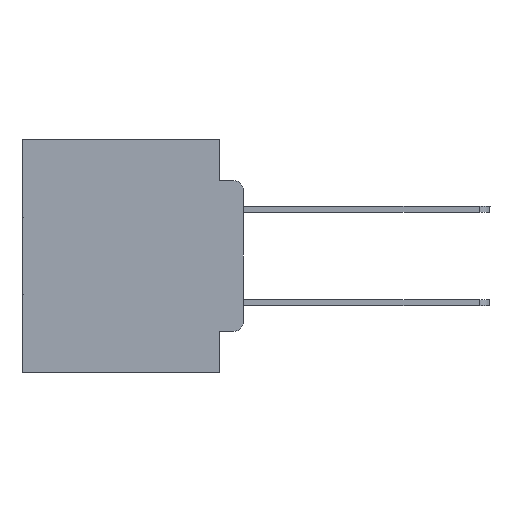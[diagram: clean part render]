
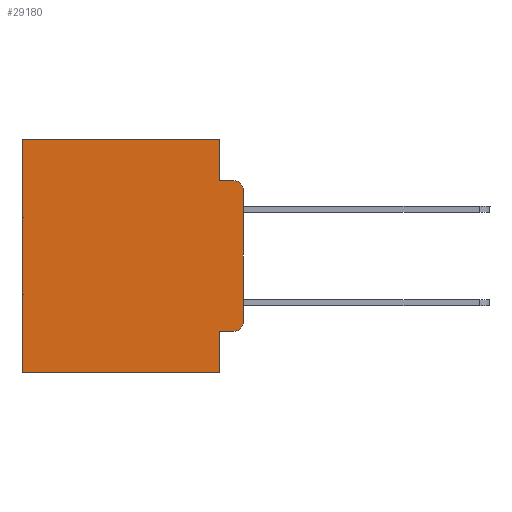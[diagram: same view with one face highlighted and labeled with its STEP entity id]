
A CAD part, left-side view. The second image highlights one B-rep face of the part: STEP entity #29180.
In plain terms, the highlighted planar face has unit normal (-1, 0, 0).
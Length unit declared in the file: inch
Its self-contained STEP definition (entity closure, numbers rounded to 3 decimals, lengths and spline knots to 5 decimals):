
#58 = DIRECTION ( 'NONE',  ( 0., 0., -1. ) ) ;
#257 = DIRECTION ( 'NONE',  ( 0., 1., 0. ) ) ;
#299 = ORIENTED_EDGE ( 'NONE', *, *, #24227, .F. ) ;
#1628 = CARTESIAN_POINT ( 'NONE',  ( 0.298, 0.02, -0.1085 ) ) ;
#1682 = CARTESIAN_POINT ( 'NONE',  ( 0.298, 0.051, 0. ) ) ;
#1748 = CARTESIAN_POINT ( 'NONE',  ( 0.298, 0., 0. ) ) ;
#1788 = VERTEX_POINT ( 'NONE', #27223 ) ;
#1991 = AXIS2_PLACEMENT_3D ( 'NONE', #17054, #2778, #19392 ) ;
#2778 = DIRECTION ( 'NONE',  ( 1., 0., 0. ) ) ;
#2850 = EDGE_CURVE ( 'NONE', #10158, #25653, #5569, .T. ) ;
#3257 = CARTESIAN_POINT ( 'NONE',  ( 0.298, 0.051, 0. ) ) ;
#3465 = ORIENTED_EDGE ( 'NONE', *, *, #28963, .T. ) ;
#3850 = VECTOR ( 'NONE', #14404, 39.37008 ) ;
#4070 = DIRECTION ( 'NONE',  ( 0., 0., -1. ) ) ;
#4407 = LINE ( 'NONE', #3257, #10001 ) ;
#4523 = ORIENTED_EDGE ( 'NONE', *, *, #12392, .T. ) ;
#4954 = EDGE_CURVE ( 'NONE', #16373, #14156, #12520, .T. ) ;
#5569 = LINE ( 'NONE', #10298, #28255 ) ;
#6296 = VERTEX_POINT ( 'NONE', #1682 ) ;
#6715 = FACE_OUTER_BOUND ( 'NONE', #25470, .T. ) ;
#7340 = VECTOR ( 'NONE', #257, 39.37008 ) ;
#9266 = CARTESIAN_POINT ( 'NONE',  ( 0.298, 0.473, -0.5 ) ) ;
#10001 = VECTOR ( 'NONE', #15132, 39.37008 ) ;
#10158 = VERTEX_POINT ( 'NONE', #15834 ) ;
#10298 = CARTESIAN_POINT ( 'NONE',  ( 0.298, 0., -0.5 ) ) ;
#10352 = AXIS2_PLACEMENT_3D ( 'NONE', #1628, #18269, #4070 ) ;
#10503 = VERTEX_POINT ( 'NONE', #22981 ) ;
#10526 = CIRCLE ( 'NONE', #27108, 0.02 ) ;
#11140 = VERTEX_POINT ( 'NONE', #15995 ) ;
#11297 = CARTESIAN_POINT ( 'NONE',  ( 0.298, 0.02, -0.0885 ) ) ;
#11565 = CARTESIAN_POINT ( 'NONE',  ( 0.298, 0.02, -0.3915 ) ) ;
#11865 = VECTOR ( 'NONE', #16343, 39.37008 ) ;
#12013 = CARTESIAN_POINT ( 'NONE',  ( 0.298, 0.051, -0.0885 ) ) ;
#12392 = EDGE_CURVE ( 'NONE', #1788, #14156, #10526, .T. ) ;
#12520 = LINE ( 'NONE', #1748, #23510 ) ;
#13088 = ORIENTED_EDGE ( 'NONE', *, *, #21128, .F. ) ;
#13953 = DIRECTION ( 'NONE',  ( 0., 0., -1. ) ) ;
#13965 = CARTESIAN_POINT ( 'NONE',  ( 0.298, 0.473, 0. ) ) ;
#14156 = VERTEX_POINT ( 'NONE', #27448 ) ;
#14404 = DIRECTION ( 'NONE',  ( 0., -1., 0. ) ) ;
#14896 = VERTEX_POINT ( 'NONE', #11297 ) ;
#14963 = ORIENTED_EDGE ( 'NONE', *, *, #22366, .T. ) ;
#15132 = DIRECTION ( 'NONE',  ( 0., 0., -1. ) ) ;
#15834 = CARTESIAN_POINT ( 'NONE',  ( 0.298, 0.051, -0.5 ) ) ;
#15995 = CARTESIAN_POINT ( 'NONE',  ( 0.298, 0.473, 0. ) ) ;
#16033 = ORIENTED_EDGE ( 'NONE', *, *, #23197, .T. ) ;
#16343 = DIRECTION ( 'NONE',  ( 0., 0., -1. ) ) ;
#16373 = VERTEX_POINT ( 'NONE', #27255 ) ;
#17054 = CARTESIAN_POINT ( 'NONE',  ( 0.298, 0., 0. ) ) ;
#17141 = ORIENTED_EDGE ( 'NONE', *, *, #18515, .F. ) ;
#17356 = LINE ( 'NONE', #19565, #28956 ) ;
#17665 = CARTESIAN_POINT ( 'NONE',  ( 0.298, 0.051, -0.4115 ) ) ;
#17792 = VERTEX_POINT ( 'NONE', #28579 ) ;
#18269 = DIRECTION ( 'NONE',  ( -1., 0., 0. ) ) ;
#18515 = EDGE_CURVE ( 'NONE', #17792, #10158, #17356, .T. ) ;
#19124 = LINE ( 'NONE', #21671, #7340 ) ;
#19296 = PLANE ( 'NONE',  #1991 ) ;
#19392 = DIRECTION ( 'NONE',  ( 0., 0., -1. ) ) ;
#19565 = CARTESIAN_POINT ( 'NONE',  ( 0.298, 0.051, 0. ) ) ;
#20011 = DIRECTION ( 'NONE',  ( 0., -1., 0. ) ) ;
#21128 = EDGE_CURVE ( 'NONE', #6296, #10503, #4407, .T. ) ;
#21671 = CARTESIAN_POINT ( 'NONE',  ( 0.298, 0., 0. ) ) ;
#21901 = DIRECTION ( 'NONE',  ( 0., 0., -1. ) ) ;
#22366 = EDGE_CURVE ( 'NONE', #6296, #11140, #19124, .T. ) ;
#22751 = LINE ( 'NONE', #17665, #26651 ) ;
#22981 = CARTESIAN_POINT ( 'NONE',  ( 0.298, 0.051, -0.0885 ) ) ;
#23197 = EDGE_CURVE ( 'NONE', #17792, #1788, #22751, .T. ) ;
#23510 = VECTOR ( 'NONE', #58, 39.37008 ) ;
#23727 = CIRCLE ( 'NONE', #10352, 0.02 ) ;
#24227 = EDGE_CURVE ( 'NONE', #10503, #14896, #29548, .T. ) ;
#24848 = EDGE_CURVE ( 'NONE', #16373, #14896, #23727, .T. ) ;
#25470 = EDGE_LOOP ( 'NONE', ( #26908, #29201, #299, #13088, #14963, #3465, #27732, #17141, #16033, #4523 ) ) ;
#25653 = VERTEX_POINT ( 'NONE', #9266 ) ;
#25850 = DIRECTION ( 'NONE',  ( 0., 1., 0. ) ) ;
#26651 = VECTOR ( 'NONE', #20011, 39.37008 ) ;
#26908 = ORIENTED_EDGE ( 'NONE', *, *, #4954, .F. ) ;
#27108 = AXIS2_PLACEMENT_3D ( 'NONE', #11565, #27870, #13953 ) ;
#27223 = CARTESIAN_POINT ( 'NONE',  ( 0.298, 0.02, -0.4115 ) ) ;
#27255 = CARTESIAN_POINT ( 'NONE',  ( 0.298, 0., -0.1085 ) ) ;
#27448 = CARTESIAN_POINT ( 'NONE',  ( 0.298, 0., -0.3915 ) ) ;
#27732 = ORIENTED_EDGE ( 'NONE', *, *, #2850, .F. ) ;
#27870 = DIRECTION ( 'NONE',  ( -1., 0., 0. ) ) ;
#28255 = VECTOR ( 'NONE', #25850, 39.37008 ) ;
#28579 = CARTESIAN_POINT ( 'NONE',  ( 0.298, 0.051, -0.4115 ) ) ;
#28956 = VECTOR ( 'NONE', #21901, 39.37008 ) ;
#28963 = EDGE_CURVE ( 'NONE', #11140, #25653, #30413, .T. ) ;
#29180 = ADVANCED_FACE ( 'NONE', ( #6715 ), #19296, .F. ) ;
#29201 = ORIENTED_EDGE ( 'NONE', *, *, #24848, .T. ) ;
#29548 = LINE ( 'NONE', #12013, #3850 ) ;
#30413 = LINE ( 'NONE', #13965, #11865 ) ;
